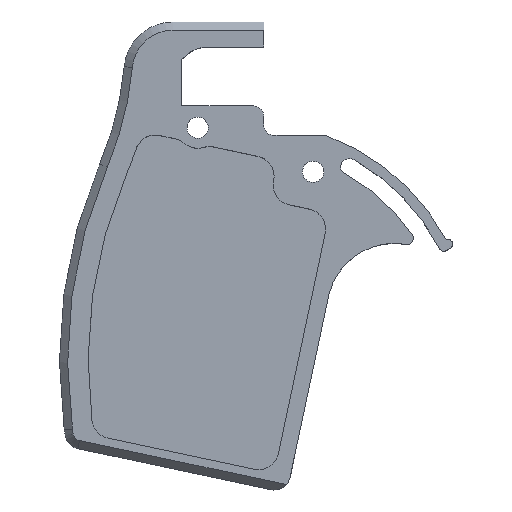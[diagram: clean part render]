
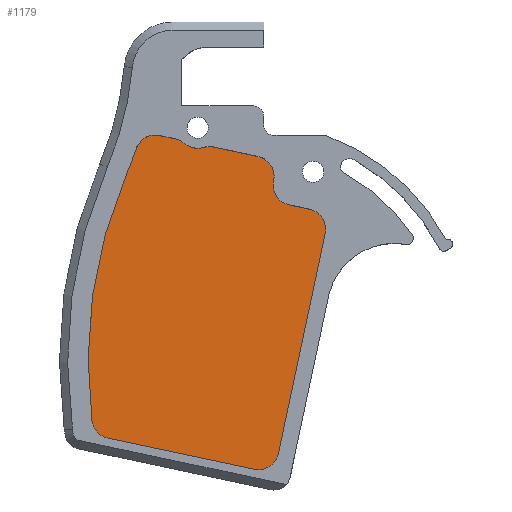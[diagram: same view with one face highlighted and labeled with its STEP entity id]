
A CAD part, top view. The second image highlights one B-rep face of the part: STEP entity #1179.
In plain terms, the highlighted planar face has unit normal (0, 0, 1).
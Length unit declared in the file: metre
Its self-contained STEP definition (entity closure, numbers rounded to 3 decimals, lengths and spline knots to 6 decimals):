
#67=CIRCLE('',#1261,0.003175);
#68=CIRCLE('',#1262,0.003175);
#69=CIRCLE('',#1263,0.003175);
#70=CIRCLE('',#1264,0.003175);
#71=CIRCLE('',#1265,0.053975);
#72=CIRCLE('',#1266,0.073025);
#73=CIRCLE('',#1267,0.003175);
#74=CIRCLE('',#1268,0.003175);
#75=CIRCLE('',#1269,0.003175);
#76=CIRCLE('',#1270,0.003175);
#77=CIRCLE('',#1271,0.003175);
#146=ORIENTED_EDGE('',*,*,#510,.F.);
#147=ORIENTED_EDGE('',*,*,#512,.T.);
#148=ORIENTED_EDGE('',*,*,#513,.F.);
#149=ORIENTED_EDGE('',*,*,#514,.T.);
#150=ORIENTED_EDGE('',*,*,#515,.F.);
#151=ORIENTED_EDGE('',*,*,#516,.T.);
#152=ORIENTED_EDGE('',*,*,#517,.F.);
#153=ORIENTED_EDGE('',*,*,#518,.F.);
#154=ORIENTED_EDGE('',*,*,#519,.T.);
#155=ORIENTED_EDGE('',*,*,#520,.T.);
#156=ORIENTED_EDGE('',*,*,#521,.T.);
#157=ORIENTED_EDGE('',*,*,#522,.F.);
#158=ORIENTED_EDGE('',*,*,#523,.T.);
#159=ORIENTED_EDGE('',*,*,#524,.F.);
#160=ORIENTED_EDGE('',*,*,#525,.T.);
#161=ORIENTED_EDGE('',*,*,#526,.T.);
#510=EDGE_CURVE('',#693,#694,#813,.T.);
#512=EDGE_CURVE('',#693,#695,#67,.F.);
#513=EDGE_CURVE('',#696,#695,#68,.F.);
#514=EDGE_CURVE('',#696,#697,#69,.F.);
#515=EDGE_CURVE('',#698,#697,#815,.T.);
#516=EDGE_CURVE('',#698,#699,#70,.F.);
#517=EDGE_CURVE('',#700,#699,#71,.T.);
#518=EDGE_CURVE('',#701,#700,#72,.T.);
#519=EDGE_CURVE('',#701,#702,#73,.F.);
#520=EDGE_CURVE('',#702,#703,#816,.T.);
#521=EDGE_CURVE('',#703,#704,#74,.F.);
#522=EDGE_CURVE('',#705,#704,#817,.T.);
#523=EDGE_CURVE('',#705,#706,#75,.F.);
#524=EDGE_CURVE('',#707,#706,#818,.T.);
#525=EDGE_CURVE('',#707,#708,#76,.T.);
#526=EDGE_CURVE('',#708,#694,#77,.F.);
#693=VERTEX_POINT('',#1804);
#694=VERTEX_POINT('',#1806);
#695=VERTEX_POINT('',#1810);
#696=VERTEX_POINT('',#1812);
#697=VERTEX_POINT('',#1814);
#698=VERTEX_POINT('',#1816);
#699=VERTEX_POINT('',#1818);
#700=VERTEX_POINT('',#1820);
#701=VERTEX_POINT('',#1822);
#702=VERTEX_POINT('',#1824);
#703=VERTEX_POINT('',#1826);
#704=VERTEX_POINT('',#1828);
#705=VERTEX_POINT('',#1830);
#706=VERTEX_POINT('',#1832);
#707=VERTEX_POINT('',#1834);
#708=VERTEX_POINT('',#1836);
#813=LINE('',#1805,#909);
#815=LINE('',#1815,#911);
#816=LINE('',#1825,#912);
#817=LINE('',#1829,#913);
#818=LINE('',#1833,#914);
#909=VECTOR('',#1412,1.);
#911=VECTOR('',#1422,1.);
#912=VECTOR('',#1431,1.);
#913=VECTOR('',#1434,1.);
#914=VECTOR('',#1437,1.);
#1004=EDGE_LOOP('',(#146,#147,#148,#149,#150,#151,#152,#153,#154,#155,#156,
#157,#158,#159,#160,#161));
#1079=FACE_BOUND('',#1004,.T.);
#1154=PLANE('',#1260);
#1179=ADVANCED_FACE('',(#1079),#1154,.F.);
#1260=AXIS2_PLACEMENT_3D('',#1808,#1414,#1415);
#1261=AXIS2_PLACEMENT_3D('',#1809,#1416,#1417);
#1262=AXIS2_PLACEMENT_3D('',#1811,#1418,#1419);
#1263=AXIS2_PLACEMENT_3D('',#1813,#1420,#1421);
#1264=AXIS2_PLACEMENT_3D('',#1817,#1423,#1424);
#1265=AXIS2_PLACEMENT_3D('',#1819,#1425,#1426);
#1266=AXIS2_PLACEMENT_3D('',#1821,#1427,#1428);
#1267=AXIS2_PLACEMENT_3D('',#1823,#1429,#1430);
#1268=AXIS2_PLACEMENT_3D('',#1827,#1432,#1433);
#1269=AXIS2_PLACEMENT_3D('',#1831,#1435,#1436);
#1270=AXIS2_PLACEMENT_3D('',#1835,#1438,#1439);
#1271=AXIS2_PLACEMENT_3D('',#1837,#1440,#1441);
#1412=DIRECTION('',(0.978,-0.208,0.));
#1414=DIRECTION('',(0.,0.,-1.));
#1415=DIRECTION('',(1.,0.,0.));
#1416=DIRECTION('',(0.,0.,-1.));
#1417=DIRECTION('',(-1.,0.,0.));
#1418=DIRECTION('',(0.,0.,-1.));
#1419=DIRECTION('',(-1.,0.,0.));
#1420=DIRECTION('',(0.,0.,-1.));
#1421=DIRECTION('',(-1.,0.,0.));
#1422=DIRECTION('',(0.978,-0.208,0.));
#1423=DIRECTION('',(0.,0.,-1.));
#1424=DIRECTION('',(-1.,0.,0.));
#1425=DIRECTION('',(0.,0.,1.));
#1426=DIRECTION('',(-1.,0.,0.));
#1427=DIRECTION('',(0.,0.,-1.));
#1428=DIRECTION('',(-1.,0.,0.));
#1429=DIRECTION('',(0.,0.,-1.));
#1430=DIRECTION('',(-1.,0.,0.));
#1431=DIRECTION('',(0.978,-0.208,0.));
#1432=DIRECTION('',(0.,0.,-1.));
#1433=DIRECTION('',(-1.,0.,0.));
#1434=DIRECTION('',(-0.208,-0.978,0.));
#1435=DIRECTION('',(0.,0.,-1.));
#1436=DIRECTION('',(-1.,0.,0.));
#1437=DIRECTION('',(0.978,-0.208,0.));
#1438=DIRECTION('',(0.,0.,-1.));
#1439=DIRECTION('',(-1.,0.,0.));
#1440=DIRECTION('',(0.,0.,-1.));
#1441=DIRECTION('',(-1.,0.,0.));
#1804=CARTESIAN_POINT('',(-0.047664,0.033473,-0.010363));
#1805=CARTESIAN_POINT('',(-0.048293,0.033607,-0.010363));
#1806=CARTESIAN_POINT('',(-0.040807,0.032015,-0.010363));
#1808=CARTESIAN_POINT('',(-0.040466,0.016342,-0.010363));
#1809=CARTESIAN_POINT('',(-0.048325,0.030367,-0.010363));
#1810=CARTESIAN_POINT('',(-0.049236,0.033409,-0.010363));
#1811=CARTESIAN_POINT('',(-0.050147,0.03645,-0.010363));
#1812=CARTESIAN_POINT('',(-0.052217,0.034042,-0.010363));
#1813=CARTESIAN_POINT('',(-0.054286,0.031635,-0.010363));
#1814=CARTESIAN_POINT('',(-0.053626,0.03474,-0.010363));
#1815=CARTESIAN_POINT('',(-0.048293,0.033607,-0.010363));
#1816=CARTESIAN_POINT('',(-0.056042,0.035254,-0.010363));
#1817=CARTESIAN_POINT('',(-0.056702,0.032148,-0.010363));
#1818=CARTESIAN_POINT('',(-0.059713,0.033158,-0.010363));
#1819=CARTESIAN_POINT('',(-0.110885,0.050324,-0.010363));
#1820=CARTESIAN_POINT('',(-0.061266,0.029081,-0.010363));
#1821=CARTESIAN_POINT('',(0.005865,0.00034,-0.010363));
#1822=CARTESIAN_POINT('',(-0.066556,-0.009031,-0.010363));
#1823=CARTESIAN_POINT('',(-0.063407,-0.008624,-0.010363));
#1824=CARTESIAN_POINT('',(-0.064067,-0.011729,-0.010363));
#1825=CARTESIAN_POINT('',(-0.050833,-0.014543,-0.010363));
#1826=CARTESIAN_POINT('',(-0.041392,-0.016549,-0.010363));
#1827=CARTESIAN_POINT('',(-0.040732,-0.013444,-0.010363));
#1828=CARTESIAN_POINT('',(-0.037626,-0.014104,-0.010363));
#1829=CARTESIAN_POINT('',(-0.03451,0.000555,-0.010363));
#1830=CARTESIAN_POINT('',(-0.030365,0.020058,-0.010363));
#1831=CARTESIAN_POINT('',(-0.03347,0.020718,-0.010363));
#1832=CARTESIAN_POINT('',(-0.03281,0.023824,-0.010363));
#1833=CARTESIAN_POINT('',(-0.042251,0.025831,-0.010363));
#1834=CARTESIAN_POINT('',(-0.035916,0.024484,-0.010363));
#1835=CARTESIAN_POINT('',(-0.035256,0.027589,-0.010363));
#1836=CARTESIAN_POINT('',(-0.038361,0.02825,-0.010363));
#1837=CARTESIAN_POINT('',(-0.041467,0.02891,-0.010363));
